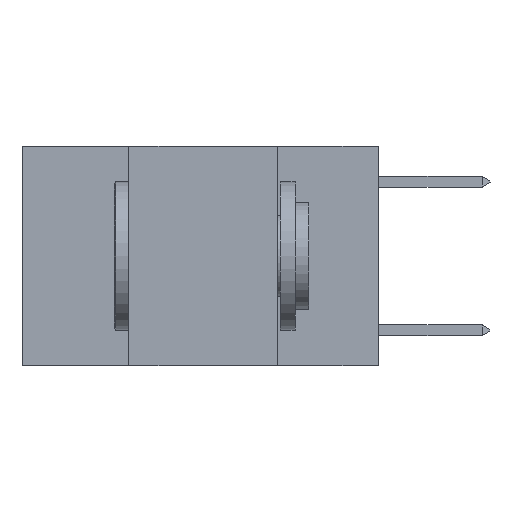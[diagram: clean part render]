
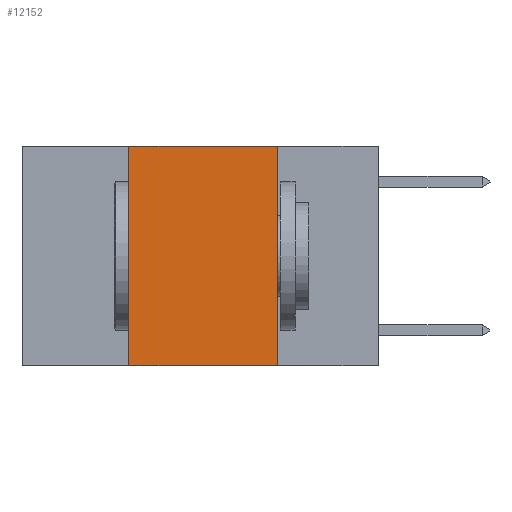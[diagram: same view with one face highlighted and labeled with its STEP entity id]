
A CAD part, left-side view. The second image highlights one B-rep face of the part: STEP entity #12152.
In plain terms, the highlighted planar face has unit normal (-1, 0, 0).
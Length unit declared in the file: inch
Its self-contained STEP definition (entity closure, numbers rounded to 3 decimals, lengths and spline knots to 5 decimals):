
#89 = DIRECTION ( 'NONE',  ( 0., 0., -1. ) ) ;
#399 = AXIS2_PLACEMENT_3D ( 'NONE', #2219, #1437, #10034 ) ;
#440 = CARTESIAN_POINT ( 'NONE',  ( 0., 0.17, -0.37 ) ) ;
#619 = VERTEX_POINT ( 'NONE', #10314 ) ;
#752 = ORIENTED_EDGE ( 'NONE', *, *, #1712, .F. ) ;
#1359 = VECTOR ( 'NONE', #89, 39.37008 ) ;
#1437 = DIRECTION ( 'NONE',  ( 1., 0., 0. ) ) ;
#1712 = EDGE_CURVE ( 'NONE', #12080, #5274, #7725, .T. ) ;
#1771 = EDGE_LOOP ( 'NONE', ( #752, #9658, #1886, #14133 ) ) ;
#1886 = ORIENTED_EDGE ( 'NONE', *, *, #12366, .F. ) ;
#2219 = CARTESIAN_POINT ( 'NONE',  ( 0., 0.6, 0. ) ) ;
#2247 = CARTESIAN_POINT ( 'NONE',  ( 0., 0.17, 0. ) ) ;
#4324 = VECTOR ( 'NONE', #12718, 39.37008 ) ;
#4325 = VECTOR ( 'NONE', #5677, 39.37008 ) ;
#4673 = CARTESIAN_POINT ( 'NONE',  ( 0., 0.6, -0.37 ) ) ;
#5271 = VECTOR ( 'NONE', #6210, 39.37008 ) ;
#5274 = VERTEX_POINT ( 'NONE', #440 ) ;
#5464 = VERTEX_POINT ( 'NONE', #8772 ) ;
#5677 = DIRECTION ( 'NONE',  ( 0., -1., 0. ) ) ;
#6210 = DIRECTION ( 'NONE',  ( 0., -1., 0. ) ) ;
#6968 = LINE ( 'NONE', #8313, #4324 ) ;
#7301 = CARTESIAN_POINT ( 'NONE',  ( 0., 0.6, 0. ) ) ;
#7725 = LINE ( 'NONE', #2247, #1359 ) ;
#8313 = CARTESIAN_POINT ( 'NONE',  ( 0., 0.42, 0. ) ) ;
#8356 = LINE ( 'NONE', #7301, #5271 ) ;
#8772 = CARTESIAN_POINT ( 'NONE',  ( 0., 0.42, 0. ) ) ;
#9034 = LINE ( 'NONE', #4673, #4325 ) ;
#9108 = PLANE ( 'NONE',  #399 ) ;
#9658 = ORIENTED_EDGE ( 'NONE', *, *, #13684, .F. ) ;
#10034 = DIRECTION ( 'NONE',  ( 0., 0., -1. ) ) ;
#10314 = CARTESIAN_POINT ( 'NONE',  ( 0., 0.42, -0.37 ) ) ;
#10684 = EDGE_CURVE ( 'NONE', #619, #5274, #9034, .T. ) ;
#11111 = CARTESIAN_POINT ( 'NONE',  ( 0., 0.17, 0. ) ) ;
#12080 = VERTEX_POINT ( 'NONE', #11111 ) ;
#12152 = ADVANCED_FACE ( 'NONE', ( #13449 ), #9108, .F. ) ;
#12366 = EDGE_CURVE ( 'NONE', #619, #5464, #6968, .T. ) ;
#12718 = DIRECTION ( 'NONE',  ( 0., 0., 1. ) ) ;
#13449 = FACE_OUTER_BOUND ( 'NONE', #1771, .T. ) ;
#13684 = EDGE_CURVE ( 'NONE', #5464, #12080, #8356, .T. ) ;
#14133 = ORIENTED_EDGE ( 'NONE', *, *, #10684, .T. ) ;
